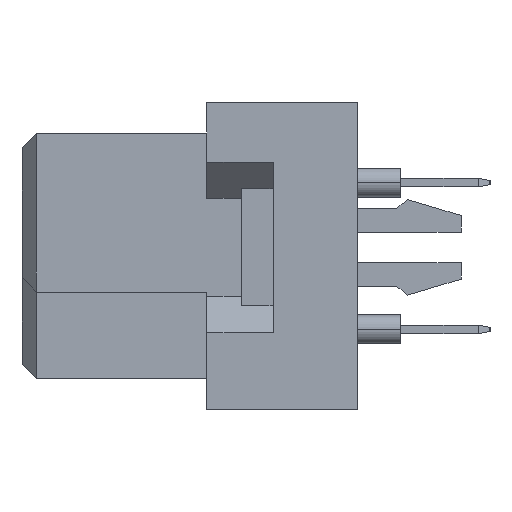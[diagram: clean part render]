
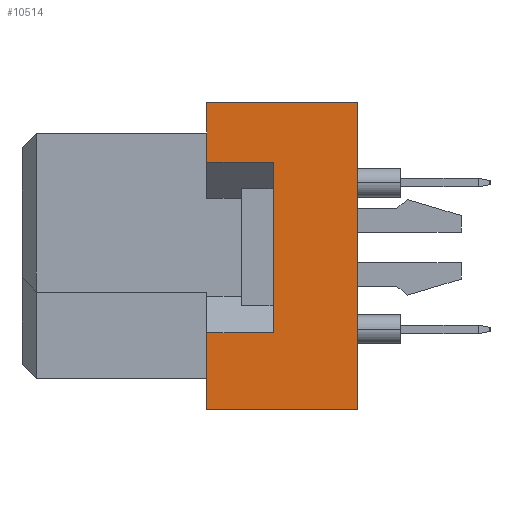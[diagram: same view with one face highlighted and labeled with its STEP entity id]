
A CAD part, left-side view. The second image highlights one B-rep face of the part: STEP entity #10514.
In plain terms, the highlighted planar face has unit normal (-1, 0, 0).
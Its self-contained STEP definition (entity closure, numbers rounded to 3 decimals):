
#34 = DIRECTION ( 'NONE',  ( 0., 0., 1. ) ) ;
#301 = EDGE_CURVE ( 'NONE', #16912, #11555, #18750, .T. ) ;
#417 = DIRECTION ( 'NONE',  ( 0., 1., 0. ) ) ;
#660 = CARTESIAN_POINT ( 'NONE',  ( -27.5, -6.4, -2.65 ) ) ;
#892 = EDGE_CURVE ( 'NONE', #16912, #8506, #20752, .T. ) ;
#1347 = EDGE_LOOP ( 'NONE', ( #6153, #5792, #18283, #11097, #3413, #5917, #12133, #11808 ) ) ;
#1749 = FACE_OUTER_BOUND ( 'NONE', #1347, .T. ) ;
#1770 = AXIS2_PLACEMENT_3D ( 'NONE', #21042, #2158, #34 ) ;
#2158 = DIRECTION ( 'NONE',  ( -1., 0., 0. ) ) ;
#2852 = CARTESIAN_POINT ( 'NONE',  ( -27.5, -6.4, -5.3 ) ) ;
#3413 = ORIENTED_EDGE ( 'NONE', *, *, #9683, .T. ) ;
#3542 = LINE ( 'NONE', #6763, #7308 ) ;
#3855 = CARTESIAN_POINT ( 'NONE',  ( -27.5, -11.6, 5.3 ) ) ;
#4294 = VECTOR ( 'NONE', #7985, 1000. ) ;
#4333 = VERTEX_POINT ( 'NONE', #660 ) ;
#4434 = CARTESIAN_POINT ( 'NONE',  ( -27.5, -6.4, 5.3 ) ) ;
#4474 = VECTOR ( 'NONE', #14464, 1000. ) ;
#5792 = ORIENTED_EDGE ( 'NONE', *, *, #12204, .F. ) ;
#5917 = ORIENTED_EDGE ( 'NONE', *, *, #14341, .F. ) ;
#6153 = ORIENTED_EDGE ( 'NONE', *, *, #9077, .T. ) ;
#6214 = DIRECTION ( 'NONE',  ( 0., 0., 1. ) ) ;
#6427 = LINE ( 'NONE', #12972, #4474 ) ;
#6763 = CARTESIAN_POINT ( 'NONE',  ( -27.5, -6.4, -5.3 ) ) ;
#6969 = CARTESIAN_POINT ( 'NONE',  ( -27.5, -11.6, -5.3 ) ) ;
#6996 = VERTEX_POINT ( 'NONE', #7563 ) ;
#7031 = CARTESIAN_POINT ( 'NONE',  ( -27.5, -11.6, 5.3 ) ) ;
#7291 = VECTOR ( 'NONE', #6214, 1000. ) ;
#7308 = VECTOR ( 'NONE', #12890, 1000. ) ;
#7508 = VERTEX_POINT ( 'NONE', #4434 ) ;
#7563 = CARTESIAN_POINT ( 'NONE',  ( -27.5, -6.4, 3.25 ) ) ;
#7985 = DIRECTION ( 'NONE',  ( 0., 0., 1. ) ) ;
#8239 = VECTOR ( 'NONE', #20951, 1000. ) ;
#8506 = VERTEX_POINT ( 'NONE', #9047 ) ;
#9047 = CARTESIAN_POINT ( 'NONE',  ( -27.5, -6.4, -5.3 ) ) ;
#9077 = EDGE_CURVE ( 'NONE', #10276, #4333, #6427, .T. ) ;
#9683 = EDGE_CURVE ( 'NONE', #11555, #7508, #13485, .T. ) ;
#10276 = VERTEX_POINT ( 'NONE', #13571 ) ;
#10514 = ADVANCED_FACE ( 'NONE', ( #1749 ), #13014, .T. ) ;
#11097 = ORIENTED_EDGE ( 'NONE', *, *, #301, .T. ) ;
#11555 = VERTEX_POINT ( 'NONE', #7031 ) ;
#11808 = ORIENTED_EDGE ( 'NONE', *, *, #15314, .F. ) ;
#12133 = ORIENTED_EDGE ( 'NONE', *, *, #13304, .F. ) ;
#12204 = EDGE_CURVE ( 'NONE', #8506, #4333, #3542, .T. ) ;
#12619 = CARTESIAN_POINT ( 'NONE',  ( -27.5, -11.6, -5.3 ) ) ;
#12890 = DIRECTION ( 'NONE',  ( 0., 0., 1. ) ) ;
#12972 = CARTESIAN_POINT ( 'NONE',  ( -27.5, -8.7, -2.65 ) ) ;
#13014 = PLANE ( 'NONE',  #1770 ) ;
#13304 = EDGE_CURVE ( 'NONE', #15753, #6996, #19751, .T. ) ;
#13426 = DIRECTION ( 'NONE',  ( 0., 1., 0. ) ) ;
#13485 = LINE ( 'NONE', #20022, #17496 ) ;
#13571 = CARTESIAN_POINT ( 'NONE',  ( -27.5, -8.7, -2.65 ) ) ;
#14341 = EDGE_CURVE ( 'NONE', #6996, #7508, #20861, .T. ) ;
#14464 = DIRECTION ( 'NONE',  ( 0., 1., 0. ) ) ;
#14565 = LINE ( 'NONE', #20889, #7291 ) ;
#15314 = EDGE_CURVE ( 'NONE', #10276, #15753, #14565, .T. ) ;
#15753 = VERTEX_POINT ( 'NONE', #17453 ) ;
#16912 = VERTEX_POINT ( 'NONE', #6969 ) ;
#17155 = DIRECTION ( 'NONE',  ( 0., 0., 1. ) ) ;
#17453 = CARTESIAN_POINT ( 'NONE',  ( -27.5, -8.7, 3.25 ) ) ;
#17496 = VECTOR ( 'NONE', #417, 1000. ) ;
#18283 = ORIENTED_EDGE ( 'NONE', *, *, #892, .F. ) ;
#18750 = LINE ( 'NONE', #3855, #21025 ) ;
#19646 = VECTOR ( 'NONE', #13426, 1000. ) ;
#19751 = LINE ( 'NONE', #19853, #19646 ) ;
#19853 = CARTESIAN_POINT ( 'NONE',  ( -27.5, -8.7, 3.25 ) ) ;
#20022 = CARTESIAN_POINT ( 'NONE',  ( -27.5, -11.6, 5.3 ) ) ;
#20752 = LINE ( 'NONE', #12619, #8239 ) ;
#20861 = LINE ( 'NONE', #2852, #4294 ) ;
#20889 = CARTESIAN_POINT ( 'NONE',  ( -27.5, -8.7, -2.65 ) ) ;
#20951 = DIRECTION ( 'NONE',  ( 0., 1., 0. ) ) ;
#21025 = VECTOR ( 'NONE', #17155, 1000. ) ;
#21042 = CARTESIAN_POINT ( 'NONE',  ( -27.5, -11.6, 5.3 ) ) ;
